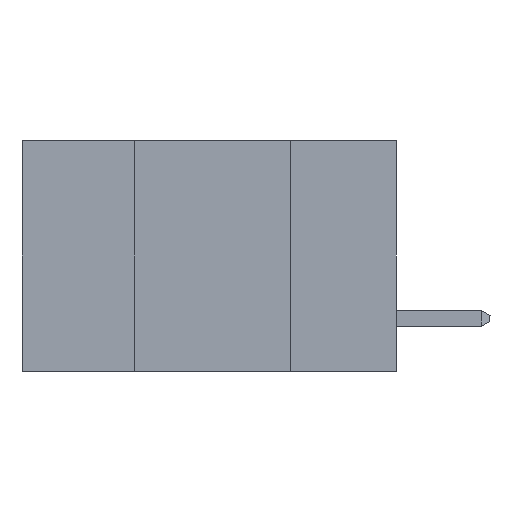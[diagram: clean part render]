
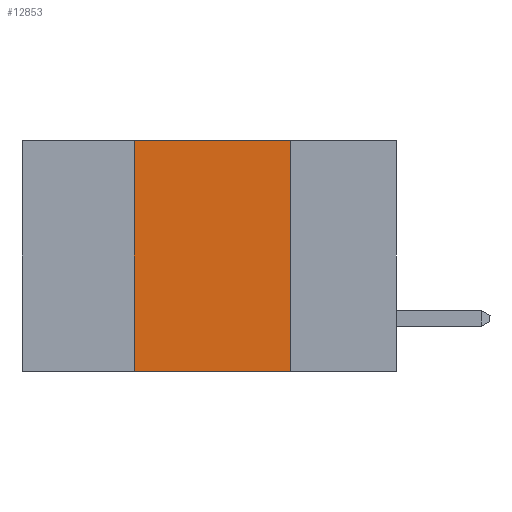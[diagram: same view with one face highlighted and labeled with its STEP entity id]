
A CAD part, left-side view. The second image highlights one B-rep face of the part: STEP entity #12853.
In plain terms, the highlighted planar face has unit normal (-1, 0, 0).
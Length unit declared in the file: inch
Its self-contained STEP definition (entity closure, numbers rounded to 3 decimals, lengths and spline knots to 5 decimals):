
#21 = VECTOR ( 'NONE', #295, 39.37008 ) ;
#242 = EDGE_CURVE ( 'NONE', #1769, #10082, #7976, .T. ) ;
#295 = DIRECTION ( 'NONE',  ( 0., 0., 1. ) ) ;
#534 = EDGE_LOOP ( 'NONE', ( #4169, #13274, #8684, #6036 ) ) ;
#910 = CARTESIAN_POINT ( 'NONE',  ( 0., 0.17, 0. ) ) ;
#1003 = CARTESIAN_POINT ( 'NONE',  ( 0., 0.6, 0. ) ) ;
#1056 = AXIS2_PLACEMENT_3D ( 'NONE', #12180, #1098, #7842 ) ;
#1076 = CARTESIAN_POINT ( 'NONE',  ( 0., 0.42, -0.37 ) ) ;
#1098 = DIRECTION ( 'NONE',  ( 1., 0., 0. ) ) ;
#1621 = EDGE_CURVE ( 'NONE', #4698, #12531, #5361, .T. ) ;
#1762 = EDGE_CURVE ( 'NONE', #10082, #4698, #8902, .T. ) ;
#1769 = VERTEX_POINT ( 'NONE', #1076 ) ;
#3774 = VECTOR ( 'NONE', #8482, 39.37008 ) ;
#4169 = ORIENTED_EDGE ( 'NONE', *, *, #1621, .F. ) ;
#4622 = LINE ( 'NONE', #9036, #7944 ) ;
#4698 = VERTEX_POINT ( 'NONE', #910 ) ;
#5361 = LINE ( 'NONE', #9768, #3774 ) ;
#5439 = DIRECTION ( 'NONE',  ( 0., -1., 0. ) ) ;
#6036 = ORIENTED_EDGE ( 'NONE', *, *, #9417, .T. ) ;
#7555 = FACE_OUTER_BOUND ( 'NONE', #534, .T. ) ;
#7842 = DIRECTION ( 'NONE',  ( 0., 0., -1. ) ) ;
#7944 = VECTOR ( 'NONE', #13423, 39.37008 ) ;
#7976 = LINE ( 'NONE', #12374, #21 ) ;
#8482 = DIRECTION ( 'NONE',  ( 0., 0., -1. ) ) ;
#8684 = ORIENTED_EDGE ( 'NONE', *, *, #242, .F. ) ;
#8902 = LINE ( 'NONE', #1003, #13557 ) ;
#9036 = CARTESIAN_POINT ( 'NONE',  ( 0., 0.6, -0.37 ) ) ;
#9417 = EDGE_CURVE ( 'NONE', #1769, #12531, #4622, .T. ) ;
#9768 = CARTESIAN_POINT ( 'NONE',  ( 0., 0.17, -0.37 ) ) ;
#10082 = VERTEX_POINT ( 'NONE', #12835 ) ;
#10942 = PLANE ( 'NONE',  #1056 ) ;
#11528 = CARTESIAN_POINT ( 'NONE',  ( 0., 0.17, -0.37 ) ) ;
#12180 = CARTESIAN_POINT ( 'NONE',  ( 0., 0.6, 0. ) ) ;
#12374 = CARTESIAN_POINT ( 'NONE',  ( 0., 0.42, -0.37 ) ) ;
#12531 = VERTEX_POINT ( 'NONE', #11528 ) ;
#12835 = CARTESIAN_POINT ( 'NONE',  ( 0., 0.42, 0. ) ) ;
#12853 = ADVANCED_FACE ( 'NONE', ( #7555 ), #10942, .F. ) ;
#13274 = ORIENTED_EDGE ( 'NONE', *, *, #1762, .F. ) ;
#13423 = DIRECTION ( 'NONE',  ( 0., -1., 0. ) ) ;
#13557 = VECTOR ( 'NONE', #5439, 39.37008 ) ;
